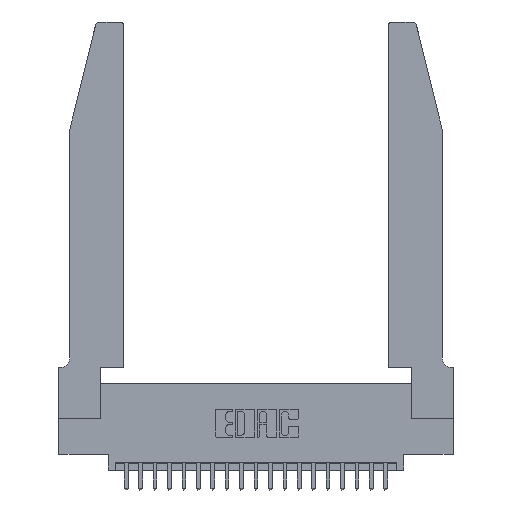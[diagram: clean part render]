
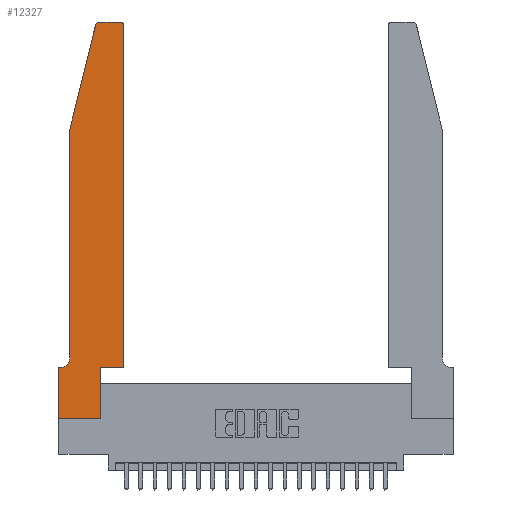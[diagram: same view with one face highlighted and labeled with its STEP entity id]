
A CAD part, top view. The second image highlights one B-rep face of the part: STEP entity #12327.
In plain terms, the highlighted planar face has unit normal (0, 0, 1).
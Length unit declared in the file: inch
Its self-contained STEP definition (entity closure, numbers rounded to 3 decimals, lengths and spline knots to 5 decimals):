
#40 = LINE ( 'NONE', #4769, #9648 ) ;
#128 = CIRCLE ( 'NONE', #12455, 0.07 ) ;
#283 = LINE ( 'NONE', #6030, #14002 ) ;
#515 = CARTESIAN_POINT ( 'NONE',  ( 0., 0.35, 0.37 ) ) ;
#552 = CARTESIAN_POINT ( 'NONE',  ( 0.25487, 2.72718, 0.37 ) ) ;
#679 = VECTOR ( 'NONE', #2092, 39.37008 ) ;
#1358 = CARTESIAN_POINT ( 'NONE',  ( 0.284, 2.75, 0.37 ) ) ;
#1838 = LINE ( 'NONE', #8029, #15523 ) ;
#1997 = VECTOR ( 'NONE', #21718, 39.37008 ) ;
#2092 = DIRECTION ( 'NONE',  ( 0., -1., 0. ) ) ;
#2223 = DIRECTION ( 'NONE',  ( 0., 1., 0. ) ) ;
#2289 = VERTEX_POINT ( 'NONE', #2790 ) ;
#2333 = DIRECTION ( 'NONE',  ( 1., 0., 0. ) ) ;
#2697 = CARTESIAN_POINT ( 'NONE',  ( 0.0755, 2., 0.37 ) ) ;
#2790 = CARTESIAN_POINT ( 'NONE',  ( 0.4505, 2.72, 0.37 ) ) ;
#3053 = CARTESIAN_POINT ( 'NONE',  ( 0.2605, 2.75, 0.37 ) ) ;
#3588 = ORIENTED_EDGE ( 'NONE', *, *, #5705, .T. ) ;
#3894 = CARTESIAN_POINT ( 'NONE',  ( 0.0755, 2., 0.37 ) ) ;
#3928 = CARTESIAN_POINT ( 'NONE',  ( 0.0055, 0.35, 0.37 ) ) ;
#4017 = EDGE_CURVE ( 'NONE', #18569, #20681, #1838, .T. ) ;
#4121 = EDGE_CURVE ( 'NONE', #9373, #22459, #128, .T. ) ;
#4669 = AXIS2_PLACEMENT_3D ( 'NONE', #17273, #6663, #18988 ) ;
#4744 = DIRECTION ( 'NONE',  ( 0., 0., -1. ) ) ;
#4769 = CARTESIAN_POINT ( 'NONE',  ( 0.0755, 0.35, 0.37 ) ) ;
#5228 = VECTOR ( 'NONE', #17289, 39.37008 ) ;
#5463 = CARTESIAN_POINT ( 'NONE',  ( 0.4505, 0.35, 0.37 ) ) ;
#5705 = EDGE_CURVE ( 'NONE', #6794, #9373, #7487, .T. ) ;
#5723 = DIRECTION ( 'NONE',  ( 0., -1., 0. ) ) ;
#6030 = CARTESIAN_POINT ( 'NONE',  ( 0.2865, 0.35, 0.37 ) ) ;
#6222 = DIRECTION ( 'NONE',  ( 1., 0., 0. ) ) ;
#6283 = DIRECTION ( 'NONE',  ( 0., 0., 1. ) ) ;
#6373 = ORIENTED_EDGE ( 'NONE', *, *, #20339, .T. ) ;
#6560 = DIRECTION ( 'NONE',  ( -1., 0., 0. ) ) ;
#6631 = ORIENTED_EDGE ( 'NONE', *, *, #10853, .T. ) ;
#6663 = DIRECTION ( 'NONE',  ( 0., 0., 1. ) ) ;
#6794 = VERTEX_POINT ( 'NONE', #8779 ) ;
#6884 = AXIS2_PLACEMENT_3D ( 'NONE', #515, #13045, #2333 ) ;
#6977 = EDGE_CURVE ( 'NONE', #18502, #21177, #14380, .T. ) ;
#7187 = ORIENTED_EDGE ( 'NONE', *, *, #14235, .T. ) ;
#7487 = LINE ( 'NONE', #3894, #11712 ) ;
#7662 = CARTESIAN_POINT ( 'NONE',  ( 0.4505, 0.35, 0.37 ) ) ;
#7852 = EDGE_CURVE ( 'NONE', #22459, #18502, #40, .T. ) ;
#8029 = CARTESIAN_POINT ( 'NONE',  ( 0.4505, 0.35, 0.37 ) ) ;
#8127 = VECTOR ( 'NONE', #2223, 39.37008 ) ;
#8164 = EDGE_LOOP ( 'NONE', ( #20335, #11765, #6373, #3588, #16281, #11776, #22387, #12509, #7187, #14633, #11303, #6631 ) ) ;
#8365 = VERTEX_POINT ( 'NONE', #14489 ) ;
#8779 = CARTESIAN_POINT ( 'NONE',  ( 0.0755, 2., 0.37 ) ) ;
#9373 = VERTEX_POINT ( 'NONE', #14272 ) ;
#9462 = CARTESIAN_POINT ( 'NONE',  ( 0.2865, 0.35, 0.37 ) ) ;
#9520 = CARTESIAN_POINT ( 'NONE',  ( 0., 0., 0.37 ) ) ;
#9569 = LINE ( 'NONE', #2697, #18161 ) ;
#9648 = VECTOR ( 'NONE', #6560, 39.37008 ) ;
#9930 = DIRECTION ( 'NONE',  ( -0.239, -0.971, 0. ) ) ;
#10047 = EDGE_CURVE ( 'NONE', #20681, #2289, #16985, .T. ) ;
#10853 = EDGE_CURVE ( 'NONE', #2289, #11943, #15899, .T. ) ;
#11294 = CIRCLE ( 'NONE', #4669, 0.03 ) ;
#11297 = PLANE ( 'NONE',  #6884 ) ;
#11303 = ORIENTED_EDGE ( 'NONE', *, *, #10047, .T. ) ;
#11590 = LINE ( 'NONE', #9520, #1997 ) ;
#11712 = VECTOR ( 'NONE', #5723, 39.37008 ) ;
#11765 = ORIENTED_EDGE ( 'NONE', *, *, #13925, .T. ) ;
#11776 = ORIENTED_EDGE ( 'NONE', *, *, #7852, .T. ) ;
#11922 = EDGE_CURVE ( 'NONE', #11943, #18243, #13557, .T. ) ;
#11943 = VERTEX_POINT ( 'NONE', #12073 ) ;
#12073 = CARTESIAN_POINT ( 'NONE',  ( 0.4205, 2.75, 0.37 ) ) ;
#12327 = ADVANCED_FACE ( 'NONE', ( #14656 ), #11297, .T. ) ;
#12455 = AXIS2_PLACEMENT_3D ( 'NONE', #15396, #4744, #17145 ) ;
#12509 = ORIENTED_EDGE ( 'NONE', *, *, #13657, .T. ) ;
#13045 = DIRECTION ( 'NONE',  ( 0., 0., 1. ) ) ;
#13557 = LINE ( 'NONE', #3053, #5228 ) ;
#13657 = EDGE_CURVE ( 'NONE', #21177, #8365, #11590, .T. ) ;
#13925 = EDGE_CURVE ( 'NONE', #18243, #14901, #11294, .T. ) ;
#14002 = VECTOR ( 'NONE', #20079, 39.37008 ) ;
#14235 = EDGE_CURVE ( 'NONE', #8365, #18569, #283, .T. ) ;
#14272 = CARTESIAN_POINT ( 'NONE',  ( 0.0755, 0.42, 0.37 ) ) ;
#14380 = LINE ( 'NONE', #14593, #679 ) ;
#14489 = CARTESIAN_POINT ( 'NONE',  ( 0.2865, 0., 0.37 ) ) ;
#14593 = CARTESIAN_POINT ( 'NONE',  ( 0., 0., 0.37 ) ) ;
#14633 = ORIENTED_EDGE ( 'NONE', *, *, #4017, .T. ) ;
#14656 = FACE_OUTER_BOUND ( 'NONE', #8164, .T. ) ;
#14901 = VERTEX_POINT ( 'NONE', #552 ) ;
#15396 = CARTESIAN_POINT ( 'NONE',  ( 0.0055, 0.42, 0.37 ) ) ;
#15523 = VECTOR ( 'NONE', #6222, 39.37008 ) ;
#15899 = CIRCLE ( 'NONE', #21999, 0.03 ) ;
#16281 = ORIENTED_EDGE ( 'NONE', *, *, #4121, .T. ) ;
#16906 = CARTESIAN_POINT ( 'NONE',  ( 0.4205, 2.72, 0.37 ) ) ;
#16985 = LINE ( 'NONE', #7662, #8127 ) ;
#17145 = DIRECTION ( 'NONE',  ( -1., 0., 0. ) ) ;
#17273 = CARTESIAN_POINT ( 'NONE',  ( 0.284, 2.72, 0.37 ) ) ;
#17289 = DIRECTION ( 'NONE',  ( -1., 0., 0. ) ) ;
#18161 = VECTOR ( 'NONE', #9930, 39.37008 ) ;
#18243 = VERTEX_POINT ( 'NONE', #1358 ) ;
#18502 = VERTEX_POINT ( 'NONE', #19690 ) ;
#18569 = VERTEX_POINT ( 'NONE', #9462 ) ;
#18632 = DIRECTION ( 'NONE',  ( 1., 0., 0. ) ) ;
#18988 = DIRECTION ( 'NONE',  ( 1., 0., 0. ) ) ;
#19512 = CARTESIAN_POINT ( 'NONE',  ( 0., 0., 0.37 ) ) ;
#19690 = CARTESIAN_POINT ( 'NONE',  ( 0., 0.35, 0.37 ) ) ;
#20079 = DIRECTION ( 'NONE',  ( 0., 1., 0. ) ) ;
#20335 = ORIENTED_EDGE ( 'NONE', *, *, #11922, .T. ) ;
#20339 = EDGE_CURVE ( 'NONE', #14901, #6794, #9569, .T. ) ;
#20681 = VERTEX_POINT ( 'NONE', #5463 ) ;
#21177 = VERTEX_POINT ( 'NONE', #19512 ) ;
#21718 = DIRECTION ( 'NONE',  ( 1., 0., 0. ) ) ;
#21999 = AXIS2_PLACEMENT_3D ( 'NONE', #16906, #6283, #18632 ) ;
#22387 = ORIENTED_EDGE ( 'NONE', *, *, #6977, .T. ) ;
#22459 = VERTEX_POINT ( 'NONE', #3928 ) ;
